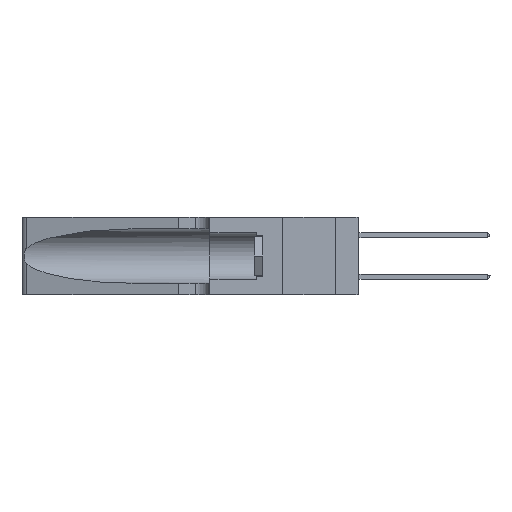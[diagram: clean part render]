
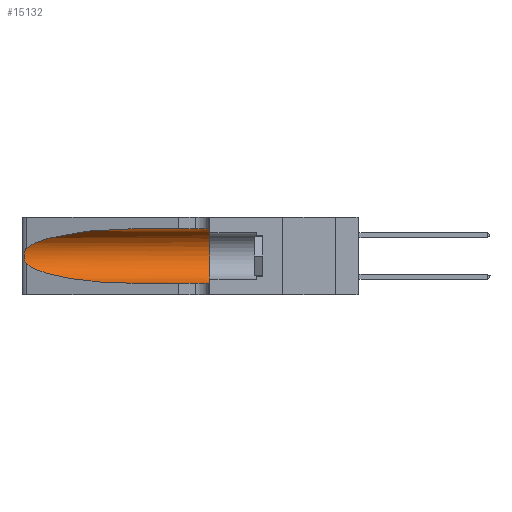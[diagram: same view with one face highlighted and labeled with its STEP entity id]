
A CAD part, left-side view. The second image highlights one B-rep face of the part: STEP entity #15132.
In plain terms, the highlighted cylindrical face has radius 3.308 mm (diameter 6.617 mm), a partial arc.
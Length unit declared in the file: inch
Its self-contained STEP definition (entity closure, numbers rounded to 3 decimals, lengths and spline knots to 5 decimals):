
#377 = VECTOR ( 'NONE', #19394, 39.37008 ) ;
#466 = CARTESIAN_POINT ( 'NONE',  ( 0.1305, 0.72297, 0.05475 ) ) ;
#1060 =( BOUNDED_CURVE ( )  B_SPLINE_CURVE ( 3, ( #6160, #6328, #20216, #466 ),
 .UNSPECIFIED., .F., .F. ) 
 B_SPLINE_CURVE_WITH_KNOTS ( ( 4, 4 ),
 ( 3.44316, 4.71239 ),
 .UNSPECIFIED. ) 
 CURVE ( )  GEOMETRIC_REPRESENTATION_ITEM ( )  RATIONAL_B_SPLINE_CURVE ( ( 1., 0.87, 0.87, 1. ) ) 
 REPRESENTATION_ITEM ( '' )  );
#1340 = VERTEX_POINT ( 'NONE', #22279 ) ;
#1426 = ORIENTED_EDGE ( 'NONE', *, *, #18756, .T. ) ;
#1653 = CARTESIAN_POINT ( 'NONE',  ( 0.1305, 1.61858, 0.31525 ) ) ;
#1968 = CARTESIAN_POINT ( 'NONE',  ( 0.25854, 1.2359, 0.20912 ) ) ;
#2208 = ORIENTED_EDGE ( 'NONE', *, *, #3799, .F. ) ;
#2398 = CARTESIAN_POINT ( 'NONE',  ( 0.1305, 1.61858, 0.05475 ) ) ;
#3213 = CYLINDRICAL_SURFACE ( 'NONE', #17410, 0.13025 ) ;
#3799 = EDGE_CURVE ( 'NONE', #8808, #23213, #17338, .T. ) ;
#4179 = CARTESIAN_POINT ( 'NONE',  ( 0.25487, 1.22718, 0.22369 ) ) ;
#5520 = LINE ( 'NONE', #2398, #14765 ) ;
#6073 = CARTESIAN_POINT ( 'NONE',  ( 0.25789, 1.23486, 0.15765 ) ) ;
#6160 = CARTESIAN_POINT ( 'NONE',  ( 0.25487, 1.22718, 0.14631 ) ) ;
#6328 = CARTESIAN_POINT ( 'NONE',  ( 0.2373, 1.15595, 0.08982 ) ) ;
#7850 = FACE_OUTER_BOUND ( 'NONE', #17390, .T. ) ;
#8808 = VERTEX_POINT ( 'NONE', #19721 ) ;
#9056 = VERTEX_POINT ( 'NONE', #19340 ) ;
#9335 = AXIS2_PLACEMENT_3D ( 'NONE', #18287, #15176, #14093 ) ;
#10047 = CARTESIAN_POINT ( 'NONE',  ( 0.25487, 1.22718, 0.14631 ) ) ;
#10128 = CARTESIAN_POINT ( 'NONE',  ( 0.25856, 1.23593, 0.16098 ) ) ;
#11203 = CARTESIAN_POINT ( 'NONE',  ( 0.1305, 0.72297, 0.31525 ) ) ;
#11450 = CARTESIAN_POINT ( 'NONE',  ( 0.25487, 1.22718, 0.22369 ) ) ;
#11764 = B_SPLINE_CURVE_WITH_KNOTS ( 'NONE', 3,
 ( #4179, #22007, #23740, #18043, #1968, #15792, #11908, #15874, #17873, #10128, #6073, #23831, #23905, #10047 ),
 .UNSPECIFIED., .F., .F.,
 ( 4, 2, 2, 2, 2, 2, 4 ),
 ( 0., 0.00027, 0.00053, 0.00107, 0.0016, 0.00187, 0.00214 ),
 .UNSPECIFIED. ) ;
#11908 = CARTESIAN_POINT ( 'NONE',  ( 0.26075, 1.23896, 0.19203 ) ) ;
#13197 =( BOUNDED_CURVE ( )  B_SPLINE_CURVE ( 3, ( #11203, #21118, #15175, #11450 ),
 .UNSPECIFIED., .F., .F. ) 
 B_SPLINE_CURVE_WITH_KNOTS ( ( 4, 4 ),
 ( 1.5708, 2.84003 ),
 .UNSPECIFIED. ) 
 CURVE ( )  GEOMETRIC_REPRESENTATION_ITEM ( )  RATIONAL_B_SPLINE_CURVE ( ( 1., 0.87, 0.87, 1. ) ) 
 REPRESENTATION_ITEM ( '' )  );
#13666 = DIRECTION ( 'NONE',  ( 0., 0., -1. ) ) ;
#14093 = DIRECTION ( 'NONE',  ( 0., 0., 1. ) ) ;
#14751 = EDGE_CURVE ( 'NONE', #23213, #9056, #18659, .T. ) ;
#14765 = VECTOR ( 'NONE', #15796, 39.37008 ) ;
#15132 = ADVANCED_FACE ( 'NONE', ( #7850 ), #3213, .F. ) ;
#15175 = CARTESIAN_POINT ( 'NONE',  ( 0.2373, 1.15595, 0.28018 ) ) ;
#15176 = DIRECTION ( 'NONE',  ( 0., 1., 0. ) ) ;
#15791 = VERTEX_POINT ( 'NONE', #15966 ) ;
#15792 = CARTESIAN_POINT ( 'NONE',  ( 0.26018, 1.23835, 0.19895 ) ) ;
#15796 = DIRECTION ( 'NONE',  ( 0., -1., 0. ) ) ;
#15874 = CARTESIAN_POINT ( 'NONE',  ( 0.26075, 1.23896, 0.178 ) ) ;
#15966 = CARTESIAN_POINT ( 'NONE',  ( 0.25487, 1.22718, 0.22369 ) ) ;
#16425 = CARTESIAN_POINT ( 'NONE',  ( 0.1305, 0.35, 0.31525 ) ) ;
#16820 = EDGE_CURVE ( 'NONE', #1340, #17206, #1060, .T. ) ;
#17206 = VERTEX_POINT ( 'NONE', #23467 ) ;
#17338 = LINE ( 'NONE', #1653, #377 ) ;
#17390 = EDGE_LOOP ( 'NONE', ( #25426, #22073, #21166, #1426, #21382, #2208 ) ) ;
#17410 = AXIS2_PLACEMENT_3D ( 'NONE', #23506, #25489, #13666 ) ;
#17873 = CARTESIAN_POINT ( 'NONE',  ( 0.26017, 1.23833, 0.17102 ) ) ;
#18043 = CARTESIAN_POINT ( 'NONE',  ( 0.25787, 1.23484, 0.2124 ) ) ;
#18287 = CARTESIAN_POINT ( 'NONE',  ( 0.1305, 0.35, 0.185 ) ) ;
#18659 = CIRCLE ( 'NONE', #9335, 0.13025 ) ;
#18756 = EDGE_CURVE ( 'NONE', #17206, #9056, #5520, .T. ) ;
#19340 = CARTESIAN_POINT ( 'NONE',  ( 0.1305, 0.35, 0.05475 ) ) ;
#19394 = DIRECTION ( 'NONE',  ( 0., -1., 0. ) ) ;
#19721 = CARTESIAN_POINT ( 'NONE',  ( 0.1305, 0.72297, 0.31525 ) ) ;
#20216 = CARTESIAN_POINT ( 'NONE',  ( 0.18966, 0.96281, 0.05475 ) ) ;
#21118 = CARTESIAN_POINT ( 'NONE',  ( 0.18966, 0.96281, 0.31525 ) ) ;
#21166 = ORIENTED_EDGE ( 'NONE', *, *, #16820, .T. ) ;
#21382 = ORIENTED_EDGE ( 'NONE', *, *, #14751, .F. ) ;
#22007 = CARTESIAN_POINT ( 'NONE',  ( 0.25555, 1.22994, 0.2215 ) ) ;
#22073 = ORIENTED_EDGE ( 'NONE', *, *, #23598, .T. ) ;
#22279 = CARTESIAN_POINT ( 'NONE',  ( 0.25487, 1.22718, 0.14631 ) ) ;
#23213 = VERTEX_POINT ( 'NONE', #16425 ) ;
#23467 = CARTESIAN_POINT ( 'NONE',  ( 0.1305, 0.72297, 0.05475 ) ) ;
#23506 = CARTESIAN_POINT ( 'NONE',  ( 0.1305, 1.61858, 0.185 ) ) ;
#23598 = EDGE_CURVE ( 'NONE', #15791, #1340, #11764, .T. ) ;
#23740 = CARTESIAN_POINT ( 'NONE',  ( 0.25639, 1.23184, 0.21858 ) ) ;
#23831 = CARTESIAN_POINT ( 'NONE',  ( 0.25639, 1.23186, 0.15144 ) ) ;
#23905 = CARTESIAN_POINT ( 'NONE',  ( 0.25555, 1.22993, 0.14849 ) ) ;
#24469 = EDGE_CURVE ( 'NONE', #8808, #15791, #13197, .T. ) ;
#25426 = ORIENTED_EDGE ( 'NONE', *, *, #24469, .T. ) ;
#25489 = DIRECTION ( 'NONE',  ( 0., -1., 0. ) ) ;
